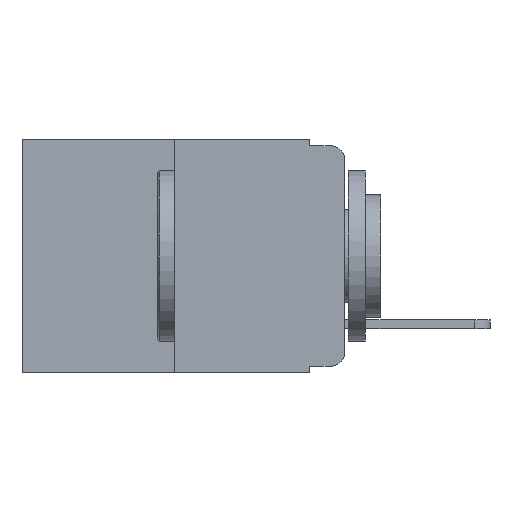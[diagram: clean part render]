
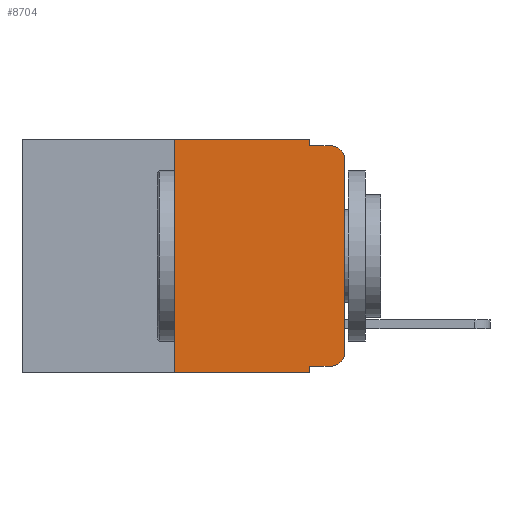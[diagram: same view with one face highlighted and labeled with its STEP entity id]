
A CAD part, left-side view. The second image highlights one B-rep face of the part: STEP entity #8704.
In plain terms, the highlighted planar face has unit normal (-1, 0, 0).
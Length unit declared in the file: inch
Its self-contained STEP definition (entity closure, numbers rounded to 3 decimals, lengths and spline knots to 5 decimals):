
#310 = CIRCLE ( 'NONE', #311, 0.02 ) ;
#311 = AXIS2_PLACEMENT_3D ( 'NONE', #1522, #12459, #3162 ) ;
#571 = ORIENTED_EDGE ( 'NONE', *, *, #18626, .F. ) ;
#866 = CARTESIAN_POINT ( 'NONE',  ( 0., 0.02, -0.333 ) ) ;
#1322 = CARTESIAN_POINT ( 'NONE',  ( 0., 0., -0.03 ) ) ;
#1350 = EDGE_CURVE ( 'NONE', #7344, #14973, #5037, .T. ) ;
#1374 = CARTESIAN_POINT ( 'NONE',  ( 0., 0.02, -0.01 ) ) ;
#1388 = PLANE ( 'NONE',  #16013 ) ;
#1498 = VERTEX_POINT ( 'NONE', #4198 ) ;
#1522 = CARTESIAN_POINT ( 'NONE',  ( 0., 0.02, -0.03 ) ) ;
#2492 = EDGE_CURVE ( 'NONE', #14973, #17331, #2558, .T. ) ;
#2558 = CIRCLE ( 'NONE', #13913, 0.02 ) ;
#2652 = VECTOR ( 'NONE', #5543, 39.37008 ) ;
#3030 = DIRECTION ( 'NONE',  ( 0., 0., -1. ) ) ;
#3162 = DIRECTION ( 'NONE',  ( 0., 0., -1. ) ) ;
#3478 = LINE ( 'NONE', #13154, #7638 ) ;
#3649 = EDGE_CURVE ( 'NONE', #4646, #9391, #13232, .T. ) ;
#3729 = CARTESIAN_POINT ( 'NONE',  ( 0., 0.051, -0.01 ) ) ;
#3859 = ORIENTED_EDGE ( 'NONE', *, *, #3649, .F. ) ;
#3868 = DIRECTION ( 'NONE',  ( 0., 0., -1. ) ) ;
#4055 = LINE ( 'NONE', #18272, #15382 ) ;
#4073 = EDGE_CURVE ( 'NONE', #6326, #4646, #13692, .T. ) ;
#4198 = CARTESIAN_POINT ( 'NONE',  ( 0., 0.051, -0.343 ) ) ;
#4287 = CARTESIAN_POINT ( 'NONE',  ( 0., 0.051, -0.333 ) ) ;
#4646 = VERTEX_POINT ( 'NONE', #14582 ) ;
#5037 = LINE ( 'NONE', #4287, #17268 ) ;
#5543 = DIRECTION ( 'NONE',  ( 0., 0., 1. ) ) ;
#5895 = VERTEX_POINT ( 'NONE', #14919 ) ;
#6326 = VERTEX_POINT ( 'NONE', #12960 ) ;
#6518 = DIRECTION ( 'NONE',  ( -1., 0., 0. ) ) ;
#6824 = LINE ( 'NONE', #11686, #19389 ) ;
#7344 = VERTEX_POINT ( 'NONE', #8752 ) ;
#7638 = VECTOR ( 'NONE', #3868, 39.37008 ) ;
#7855 = EDGE_CURVE ( 'NONE', #17331, #12697, #10955, .T. ) ;
#8704 = ADVANCED_FACE ( 'NONE', ( #15882 ), #1388, .F. ) ;
#8752 = CARTESIAN_POINT ( 'NONE',  ( 0., 0.051, -0.333 ) ) ;
#9167 = VECTOR ( 'NONE', #13696, 39.37008 ) ;
#9210 = EDGE_CURVE ( 'NONE', #5895, #1498, #14447, .T. ) ;
#9391 = VERTEX_POINT ( 'NONE', #3729 ) ;
#9492 = ORIENTED_EDGE ( 'NONE', *, *, #2492, .T. ) ;
#9638 = VECTOR ( 'NONE', #13219, 39.37008 ) ;
#10499 = DIRECTION ( 'NONE',  ( 0., 0., -1. ) ) ;
#10793 = CARTESIAN_POINT ( 'NONE',  ( 0., 0.473, 0. ) ) ;
#10955 = LINE ( 'NONE', #17803, #2652 ) ;
#11637 = CARTESIAN_POINT ( 'NONE',  ( 0., 0., -0.313 ) ) ;
#11657 = ORIENTED_EDGE ( 'NONE', *, *, #16492, .T. ) ;
#11686 = CARTESIAN_POINT ( 'NONE',  ( 0., 0.25, 0. ) ) ;
#11698 = CARTESIAN_POINT ( 'NONE',  ( 0., 0.473, 0. ) ) ;
#12035 = CARTESIAN_POINT ( 'NONE',  ( 0., 0.473, -0.343 ) ) ;
#12125 = ORIENTED_EDGE ( 'NONE', *, *, #4073, .F. ) ;
#12329 = DIRECTION ( 'NONE',  ( 1., 0., 0. ) ) ;
#12459 = DIRECTION ( 'NONE',  ( -1., 0., 0. ) ) ;
#12604 = ORIENTED_EDGE ( 'NONE', *, *, #16182, .F. ) ;
#12697 = VERTEX_POINT ( 'NONE', #1322 ) ;
#12960 = CARTESIAN_POINT ( 'NONE',  ( 0., 0.25, 0. ) ) ;
#13082 = ORIENTED_EDGE ( 'NONE', *, *, #1350, .T. ) ;
#13154 = CARTESIAN_POINT ( 'NONE',  ( 0., 0.051, 0. ) ) ;
#13207 = DIRECTION ( 'NONE',  ( 0., 0., 1. ) ) ;
#13219 = DIRECTION ( 'NONE',  ( 0., -1., 0. ) ) ;
#13232 = LINE ( 'NONE', #18135, #9167 ) ;
#13692 = LINE ( 'NONE', #11698, #9638 ) ;
#13696 = DIRECTION ( 'NONE',  ( 0., 0., -1. ) ) ;
#13913 = AXIS2_PLACEMENT_3D ( 'NONE', #14177, #6518, #10499 ) ;
#14062 = EDGE_CURVE ( 'NONE', #9391, #14091, #4055, .T. ) ;
#14091 = VERTEX_POINT ( 'NONE', #1374 ) ;
#14177 = CARTESIAN_POINT ( 'NONE',  ( 0., 0.02, -0.313 ) ) ;
#14447 = LINE ( 'NONE', #12035, #17950 ) ;
#14582 = CARTESIAN_POINT ( 'NONE',  ( 0., 0.051, 0. ) ) ;
#14919 = CARTESIAN_POINT ( 'NONE',  ( 0., 0.25, -0.343 ) ) ;
#14973 = VERTEX_POINT ( 'NONE', #866 ) ;
#15284 = DIRECTION ( 'NONE',  ( 0., -1., 0. ) ) ;
#15382 = VECTOR ( 'NONE', #15284, 39.37008 ) ;
#15657 = ORIENTED_EDGE ( 'NONE', *, *, #14062, .F. ) ;
#15882 = FACE_OUTER_BOUND ( 'NONE', #18497, .T. ) ;
#15935 = DIRECTION ( 'NONE',  ( 0., -1., 0. ) ) ;
#16013 = AXIS2_PLACEMENT_3D ( 'NONE', #10793, #12329, #3030 ) ;
#16182 = EDGE_CURVE ( 'NONE', #5895, #6326, #6824, .T. ) ;
#16492 = EDGE_CURVE ( 'NONE', #12697, #14091, #310, .T. ) ;
#16578 = DIRECTION ( 'NONE',  ( 0., -1., 0. ) ) ;
#16594 = ORIENTED_EDGE ( 'NONE', *, *, #9210, .T. ) ;
#17268 = VECTOR ( 'NONE', #15935, 39.37008 ) ;
#17331 = VERTEX_POINT ( 'NONE', #11637 ) ;
#17803 = CARTESIAN_POINT ( 'NONE',  ( 0., 0., 0. ) ) ;
#17950 = VECTOR ( 'NONE', #16578, 39.37008 ) ;
#18135 = CARTESIAN_POINT ( 'NONE',  ( 0., 0.051, 0. ) ) ;
#18272 = CARTESIAN_POINT ( 'NONE',  ( 0., 0.051, -0.01 ) ) ;
#18497 = EDGE_LOOP ( 'NONE', ( #19143, #11657, #15657, #3859, #12125, #12604, #16594, #571, #13082, #9492 ) ) ;
#18626 = EDGE_CURVE ( 'NONE', #7344, #1498, #3478, .T. ) ;
#19143 = ORIENTED_EDGE ( 'NONE', *, *, #7855, .T. ) ;
#19389 = VECTOR ( 'NONE', #13207, 39.37008 ) ;
